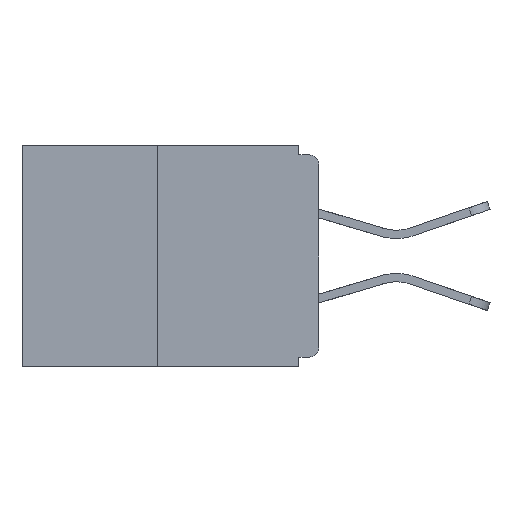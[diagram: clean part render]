
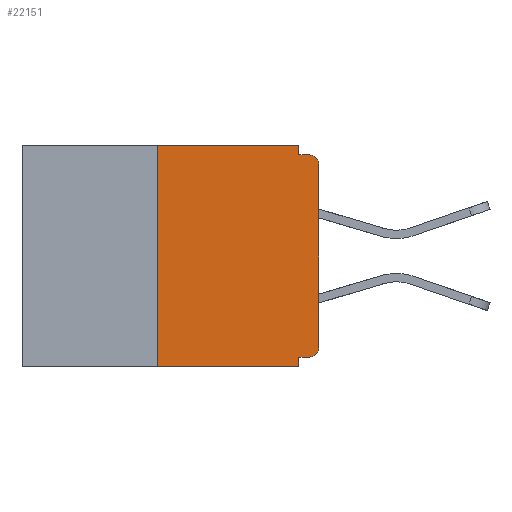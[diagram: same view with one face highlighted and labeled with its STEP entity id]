
A CAD part, left-side view. The second image highlights one B-rep face of the part: STEP entity #22151.
In plain terms, the highlighted planar face has unit normal (-1, 0, 0).
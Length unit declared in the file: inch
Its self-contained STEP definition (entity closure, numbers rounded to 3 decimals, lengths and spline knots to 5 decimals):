
#7 = VERTEX_POINT ( 'NONE', #11720 ) ;
#538 = DIRECTION ( 'NONE',  ( 0., 0., -1. ) ) ;
#710 = ORIENTED_EDGE ( 'NONE', *, *, #20871, .F. ) ;
#1525 = DIRECTION ( 'NONE',  ( 0., 0., -1. ) ) ;
#2019 = DIRECTION ( 'NONE',  ( 0., 0., -1. ) ) ;
#2951 = CARTESIAN_POINT ( 'NONE',  ( 0., 0., -0.03 ) ) ;
#3361 = AXIS2_PLACEMENT_3D ( 'NONE', #29908, #22810, #1525 ) ;
#4482 = VERTEX_POINT ( 'NONE', #29888 ) ;
#4702 = ORIENTED_EDGE ( 'NONE', *, *, #28076, .F. ) ;
#4885 = VECTOR ( 'NONE', #20214, 39.37008 ) ;
#4957 = AXIS2_PLACEMENT_3D ( 'NONE', #18824, #22960, #26072 ) ;
#5986 = CIRCLE ( 'NONE', #17552, 0.015 ) ;
#6044 = CARTESIAN_POINT ( 'NONE',  ( 0., 0., -0.328 ) ) ;
#6367 = LINE ( 'NONE', #6044, #22322 ) ;
#6519 = VERTEX_POINT ( 'NONE', #21082 ) ;
#7433 = EDGE_CURVE ( 'NONE', #10492, #31106, #15908, .T. ) ;
#8019 = DIRECTION ( 'NONE',  ( 0., -1., 0. ) ) ;
#8062 = LINE ( 'NONE', #10906, #4885 ) ;
#8225 = LINE ( 'NONE', #18153, #12815 ) ;
#8362 = DIRECTION ( 'NONE',  ( 0., 0., 1. ) ) ;
#9413 = CIRCLE ( 'NONE', #3361, 0.015 ) ;
#9516 = VERTEX_POINT ( 'NONE', #2951 ) ;
#9613 = EDGE_CURVE ( 'NONE', #24975, #11256, #9413, .T. ) ;
#10102 = VERTEX_POINT ( 'NONE', #23867 ) ;
#10390 = CARTESIAN_POINT ( 'NONE',  ( 0., 0.46, -0.343 ) ) ;
#10454 = EDGE_CURVE ( 'NONE', #7, #10492, #8062, .T. ) ;
#10475 = ORIENTED_EDGE ( 'NONE', *, *, #18222, .T. ) ;
#10492 = VERTEX_POINT ( 'NONE', #24939 ) ;
#10906 = CARTESIAN_POINT ( 'NONE',  ( 0., 0.25, 0. ) ) ;
#11068 = EDGE_LOOP ( 'NONE', ( #11657, #20118, #30230, #710, #13692, #23943, #29260, #10475, #4702, #16490 ) ) ;
#11256 = VERTEX_POINT ( 'NONE', #14072 ) ;
#11657 = ORIENTED_EDGE ( 'NONE', *, *, #7433, .F. ) ;
#11720 = CARTESIAN_POINT ( 'NONE',  ( 0., 0.25, -0.343 ) ) ;
#12815 = VECTOR ( 'NONE', #30142, 39.37008 ) ;
#13692 = ORIENTED_EDGE ( 'NONE', *, *, #25792, .F. ) ;
#13840 = DIRECTION ( 'NONE',  ( 0., -1., 0. ) ) ;
#13994 = CARTESIAN_POINT ( 'NONE',  ( 0., 0.46, 0. ) ) ;
#14003 = LINE ( 'NONE', #28514, #17682 ) ;
#14072 = CARTESIAN_POINT ( 'NONE',  ( 0., 0., -0.313 ) ) ;
#14371 = CARTESIAN_POINT ( 'NONE',  ( 0., 0.031, 0. ) ) ;
#14497 = LINE ( 'NONE', #15122, #20709 ) ;
#14916 = CARTESIAN_POINT ( 'NONE',  ( 0., 0.015, -0.03 ) ) ;
#15122 = CARTESIAN_POINT ( 'NONE',  ( 0., 0., -0.015 ) ) ;
#15908 = LINE ( 'NONE', #13994, #26024 ) ;
#16490 = ORIENTED_EDGE ( 'NONE', *, *, #27408, .F. ) ;
#16827 = CARTESIAN_POINT ( 'NONE',  ( 0., 0.015, -0.328 ) ) ;
#17552 = AXIS2_PLACEMENT_3D ( 'NONE', #14916, #24517, #538 ) ;
#17682 = VECTOR ( 'NONE', #2019, 39.37008 ) ;
#18153 = CARTESIAN_POINT ( 'NONE',  ( 0., 0.031, 0. ) ) ;
#18222 = EDGE_CURVE ( 'NONE', #9516, #20862, #5986, .T. ) ;
#18824 = CARTESIAN_POINT ( 'NONE',  ( 0., 0.46, 0. ) ) ;
#18886 = CARTESIAN_POINT ( 'NONE',  ( 0., 0.015, -0.015 ) ) ;
#19838 = DIRECTION ( 'NONE',  ( 0., -1., 0. ) ) ;
#20118 = ORIENTED_EDGE ( 'NONE', *, *, #10454, .F. ) ;
#20214 = DIRECTION ( 'NONE',  ( 0., 0., 1. ) ) ;
#20709 = VECTOR ( 'NONE', #19838, 39.37008 ) ;
#20862 = VERTEX_POINT ( 'NONE', #18886 ) ;
#20871 = EDGE_CURVE ( 'NONE', #4482, #6519, #14003, .T. ) ;
#21082 = CARTESIAN_POINT ( 'NONE',  ( 0., 0.031, -0.343 ) ) ;
#22151 = ADVANCED_FACE ( 'NONE', ( #30216 ), #27857, .F. ) ;
#22322 = VECTOR ( 'NONE', #27820, 39.37008 ) ;
#22810 = DIRECTION ( 'NONE',  ( -1., 0., 0. ) ) ;
#22960 = DIRECTION ( 'NONE',  ( 1., 0., 0. ) ) ;
#23361 = VECTOR ( 'NONE', #8362, 39.37008 ) ;
#23867 = CARTESIAN_POINT ( 'NONE',  ( 0., 0.031, -0.015 ) ) ;
#23943 = ORIENTED_EDGE ( 'NONE', *, *, #9613, .T. ) ;
#24517 = DIRECTION ( 'NONE',  ( -1., 0., 0. ) ) ;
#24939 = CARTESIAN_POINT ( 'NONE',  ( 0., 0.25, 0. ) ) ;
#24975 = VERTEX_POINT ( 'NONE', #16827 ) ;
#25284 = EDGE_CURVE ( 'NONE', #7, #6519, #30523, .T. ) ;
#25792 = EDGE_CURVE ( 'NONE', #24975, #4482, #6367, .T. ) ;
#26024 = VECTOR ( 'NONE', #13840, 39.37008 ) ;
#26072 = DIRECTION ( 'NONE',  ( 0., 0., -1. ) ) ;
#27408 = EDGE_CURVE ( 'NONE', #31106, #10102, #8225, .T. ) ;
#27775 = LINE ( 'NONE', #28090, #23361 ) ;
#27820 = DIRECTION ( 'NONE',  ( 0., 1., 0. ) ) ;
#27857 = PLANE ( 'NONE',  #4957 ) ;
#28076 = EDGE_CURVE ( 'NONE', #10102, #20862, #14497, .T. ) ;
#28090 = CARTESIAN_POINT ( 'NONE',  ( 0., 0., 0. ) ) ;
#28514 = CARTESIAN_POINT ( 'NONE',  ( 0., 0.031, -0.343 ) ) ;
#29260 = ORIENTED_EDGE ( 'NONE', *, *, #30993, .T. ) ;
#29888 = CARTESIAN_POINT ( 'NONE',  ( 0., 0.031, -0.328 ) ) ;
#29908 = CARTESIAN_POINT ( 'NONE',  ( 0., 0.015, -0.313 ) ) ;
#30142 = DIRECTION ( 'NONE',  ( 0., 0., -1. ) ) ;
#30216 = FACE_OUTER_BOUND ( 'NONE', #11068, .T. ) ;
#30230 = ORIENTED_EDGE ( 'NONE', *, *, #25284, .T. ) ;
#30353 = VECTOR ( 'NONE', #8019, 39.37008 ) ;
#30523 = LINE ( 'NONE', #10390, #30353 ) ;
#30993 = EDGE_CURVE ( 'NONE', #11256, #9516, #27775, .T. ) ;
#31106 = VERTEX_POINT ( 'NONE', #14371 ) ;
